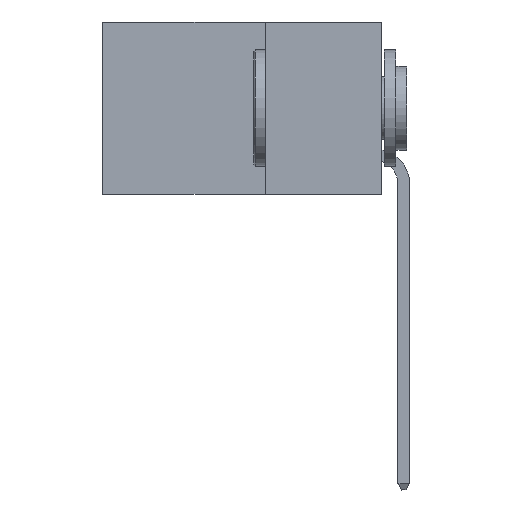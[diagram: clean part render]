
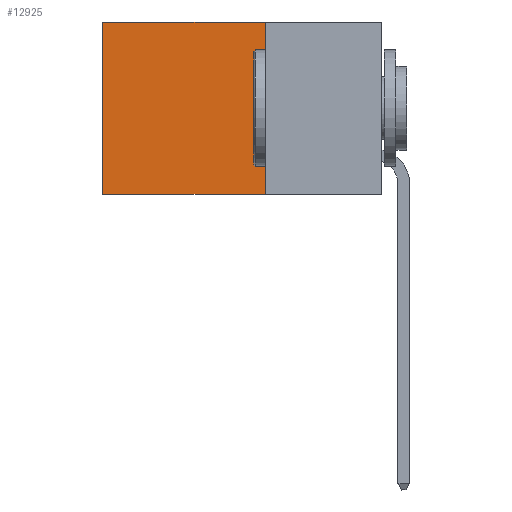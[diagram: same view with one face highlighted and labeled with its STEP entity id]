
A CAD part, left-side view. The second image highlights one B-rep face of the part: STEP entity #12925.
In plain terms, the highlighted planar face has unit normal (-1, 0, 0).
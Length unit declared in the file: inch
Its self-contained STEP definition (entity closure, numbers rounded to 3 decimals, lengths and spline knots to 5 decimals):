
#206 = CARTESIAN_POINT ( 'NONE',  ( 0.2875, 0.25, 0. ) ) ;
#2023 = VERTEX_POINT ( 'NONE', #5981 ) ;
#2069 = DIRECTION ( 'NONE',  ( 0., 0., -1. ) ) ;
#2261 = AXIS2_PLACEMENT_3D ( 'NONE', #10011, #18174, #2069 ) ;
#2697 = CARTESIAN_POINT ( 'NONE',  ( 0.2875, 0.6, 0. ) ) ;
#3708 = LINE ( 'NONE', #23963, #20787 ) ;
#5306 = EDGE_CURVE ( 'NONE', #13900, #2023, #7602, .T. ) ;
#5443 = DIRECTION ( 'NONE',  ( 0., 1., 0. ) ) ;
#5981 = CARTESIAN_POINT ( 'NONE',  ( 0.2875, 0.25, -0.37 ) ) ;
#7315 = ORIENTED_EDGE ( 'NONE', *, *, #15445, .T. ) ;
#7602 = LINE ( 'NONE', #206, #25338 ) ;
#7851 = VERTEX_POINT ( 'NONE', #20150 ) ;
#8900 = EDGE_CURVE ( 'NONE', #2023, #19539, #14015, .T. ) ;
#10011 = CARTESIAN_POINT ( 'NONE',  ( 0.2875, 0.25, 0. ) ) ;
#10275 = DIRECTION ( 'NONE',  ( 0., 0., -1. ) ) ;
#12925 = ADVANCED_FACE ( 'NONE', ( #14461 ), #24275, .F. ) ;
#13001 = VECTOR ( 'NONE', #13018, 39.37008 ) ;
#13018 = DIRECTION ( 'NONE',  ( 0., 0., -1. ) ) ;
#13900 = VERTEX_POINT ( 'NONE', #23163 ) ;
#14015 = LINE ( 'NONE', #18404, #24162 ) ;
#14126 = EDGE_CURVE ( 'NONE', #13900, #7851, #3708, .T. ) ;
#14461 = FACE_OUTER_BOUND ( 'NONE', #19245, .T. ) ;
#15445 = EDGE_CURVE ( 'NONE', #7851, #19539, #19062, .T. ) ;
#16205 = CARTESIAN_POINT ( 'NONE',  ( 0.2875, 0.6, -0.37 ) ) ;
#17570 = ORIENTED_EDGE ( 'NONE', *, *, #14126, .T. ) ;
#18174 = DIRECTION ( 'NONE',  ( 1., 0., 0. ) ) ;
#18404 = CARTESIAN_POINT ( 'NONE',  ( 0.2875, 0.25, -0.37 ) ) ;
#18640 = ORIENTED_EDGE ( 'NONE', *, *, #8900, .F. ) ;
#19062 = LINE ( 'NONE', #2697, #13001 ) ;
#19245 = EDGE_LOOP ( 'NONE', ( #7315, #18640, #22270, #17570 ) ) ;
#19539 = VERTEX_POINT ( 'NONE', #16205 ) ;
#19909 = DIRECTION ( 'NONE',  ( 0., 1., 0. ) ) ;
#20150 = CARTESIAN_POINT ( 'NONE',  ( 0.2875, 0.6, 0. ) ) ;
#20787 = VECTOR ( 'NONE', #19909, 39.37008 ) ;
#22270 = ORIENTED_EDGE ( 'NONE', *, *, #5306, .F. ) ;
#23163 = CARTESIAN_POINT ( 'NONE',  ( 0.2875, 0.25, 0. ) ) ;
#23963 = CARTESIAN_POINT ( 'NONE',  ( 0.2875, 0.25, 0. ) ) ;
#24162 = VECTOR ( 'NONE', #5443, 39.37008 ) ;
#24275 = PLANE ( 'NONE',  #2261 ) ;
#25338 = VECTOR ( 'NONE', #10275, 39.37008 ) ;
